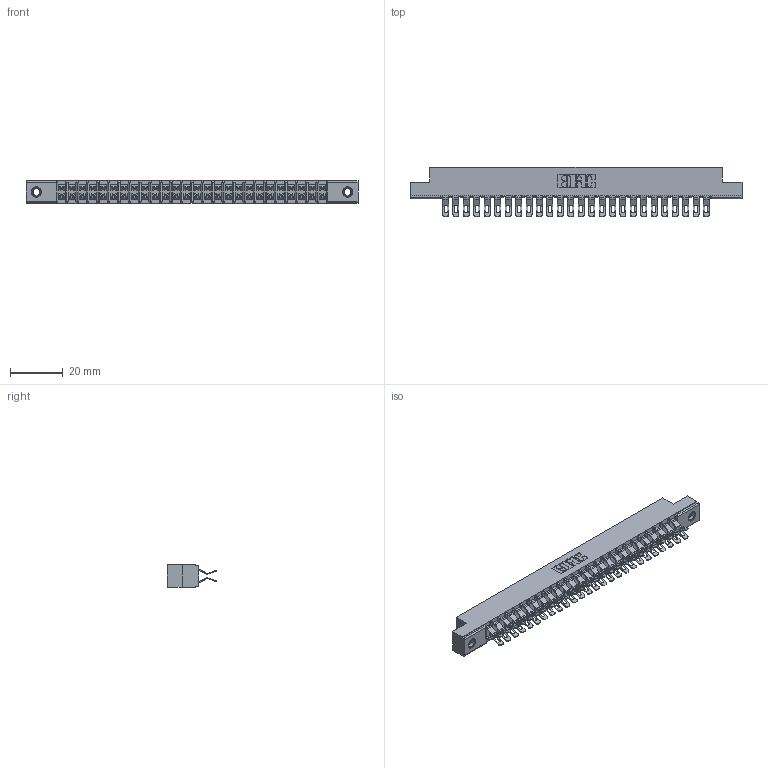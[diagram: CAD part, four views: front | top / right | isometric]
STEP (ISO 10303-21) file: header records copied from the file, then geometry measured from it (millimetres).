
FILE_DESCRIPTION (( 'STEP AP203' ), '1' );
FILE_NAME ('357-052-555-207.STEP', '2018-08-11T15:58:40', ( '' ), ( '' ), 'SwSTEP 2.0', 'SolidWorks 2016', '' );
FILE_SCHEMA (( 'CONFIG_CONTROL_DESIGN' ));
Length unit declared in the file: inch
Products named in the file (4): 345-250-001_345-250-005-103; 357-052-555-207; 307 Part_.156 Dia Mounting Holes; 307-290-001_555
Assembly tree (55 placements, depth 2):
  357-052-555-207
    307 Part_.156 Dia Mounting Holes
    307-290-001_555  x52
    345-250-001_345-250-005-103  x2
Bounding box: 126.03 x 18.75 x 8.71 mm (x, y, z)
Volume: 8385 mm3; surface area: 15912.3 mm2
Topology: 55 solids, 55 shells, 3377 faces, 9871 edges, 6430 vertices
Faces by surface type: plane 1870, cylinder 1437, sphere 54, cone 12, torus 4
Entity records: 26816 total; most frequent: CARTESIAN_POINT 4381, ORIENTED_EDGE 4336, DIRECTION 4314, EDGE_CURVE 2168, LINE 1644, VECTOR 1644, VERTEX_POINT 1402, AXIS2_PLACEMENT_3D 1335
